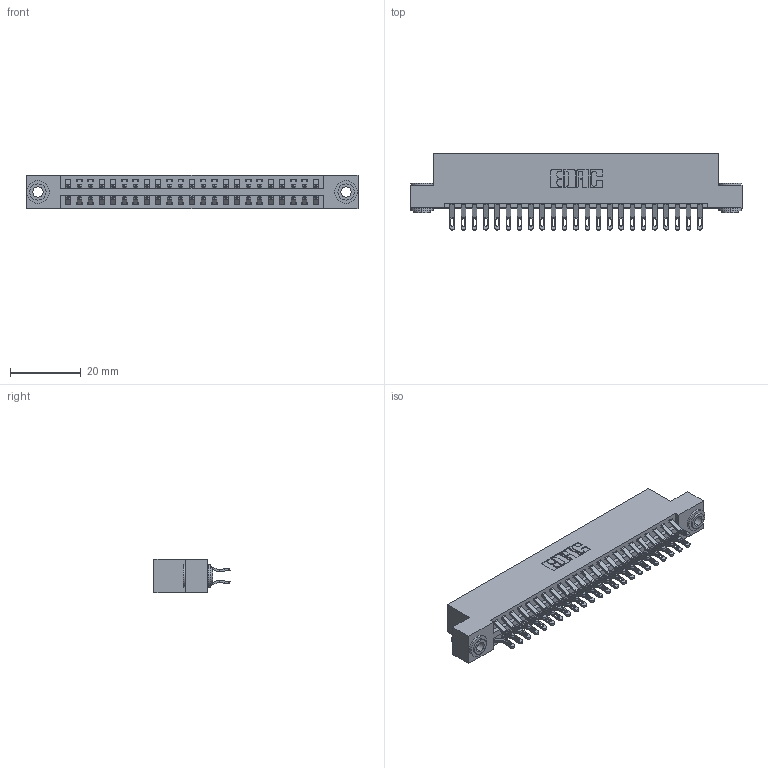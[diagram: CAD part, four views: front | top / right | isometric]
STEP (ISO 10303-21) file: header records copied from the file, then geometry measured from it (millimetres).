
FILE_DESCRIPTION (( 'STEP AP203' ), '1' );
FILE_NAME ('396-046-555-203.STEP', '2019-10-30T12:06:58', ( '' ), ( '' ), 'SwSTEP 2.0', 'SolidWorks 2016', '' );
FILE_SCHEMA (( 'CONFIG_CONTROL_DESIGN' ));
Length unit declared in the file: inch
Products named in the file (4): 346 Part_Flush Mounting Lugs - 0.156 Dia-TH; 345-250-002_345-250-002-102; 396-046-555-203; 345-292-001_555 Tail
Assembly tree (49 placements, depth 2):
  396-046-555-203
    346 Part_Flush Mounting Lugs - 0.156 Dia-TH
    345-292-001_555 Tail  x46
    345-250-002_345-250-002-102  x2
Bounding box: 93.6 x 21.46 x 9.4 mm (x, y, z)
Volume: 9132.3 mm3; surface area: 12944.1 mm2
Topology: 49 solids, 49 shells, 2828 faces, 8823 edges, 5878 vertices
Faces by surface type: plane 1604, cylinder 1216, cone 8
Entity records: 18544 total; most frequent: CARTESIAN_POINT 3093, ORIENTED_EDGE 2990, DIRECTION 2777, EDGE_CURVE 1495, LINE 1227, VECTOR 1227, VERTEX_POINT 994, AXIS2_PLACEMENT_3D 775
